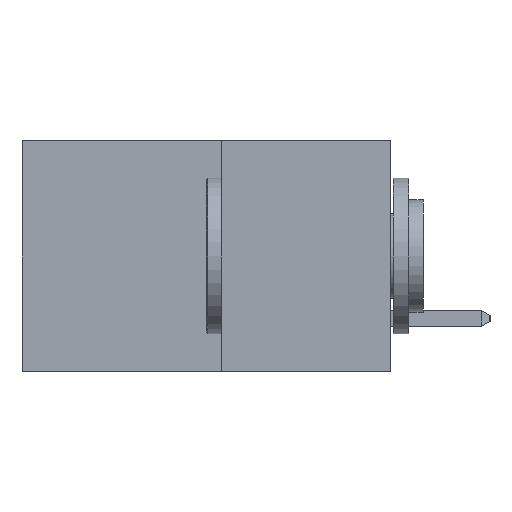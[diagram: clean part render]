
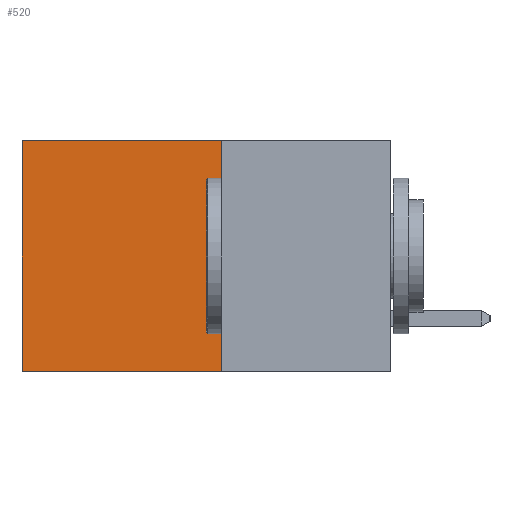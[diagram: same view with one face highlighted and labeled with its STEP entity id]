
A CAD part, left-side view. The second image highlights one B-rep face of the part: STEP entity #520.
In plain terms, the highlighted planar face has unit normal (-1, 0, 0).
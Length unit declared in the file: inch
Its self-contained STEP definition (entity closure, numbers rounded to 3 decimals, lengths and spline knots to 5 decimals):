
#131 = VERTEX_POINT ( 'NONE', #5667 ) ;
#368 = DIRECTION ( 'NONE',  ( 0., 1., 0. ) ) ;
#520 = ADVANCED_FACE ( 'NONE', ( #6625 ), #3044, .F. ) ;
#796 = ORIENTED_EDGE ( 'NONE', *, *, #4600, .F. ) ;
#2286 = DIRECTION ( 'NONE',  ( 0., 0., -1. ) ) ;
#2461 = LINE ( 'NONE', #7073, #4232 ) ;
#2730 = ORIENTED_EDGE ( 'NONE', *, *, #5847, .T. ) ;
#2867 = EDGE_LOOP ( 'NONE', ( #3276, #7098, #796, #2730 ) ) ;
#2904 = VECTOR ( 'NONE', #368, 39.37008 ) ;
#2988 = DIRECTION ( 'NONE',  ( 0., 0., -1. ) ) ;
#3044 = PLANE ( 'NONE',  #6554 ) ;
#3106 = CARTESIAN_POINT ( 'NONE',  ( 0.277, 0.59, 0. ) ) ;
#3276 = ORIENTED_EDGE ( 'NONE', *, *, #8350, .T. ) ;
#3487 = VECTOR ( 'NONE', #8264, 39.37008 ) ;
#4004 = DIRECTION ( 'NONE',  ( 1., 0., 0. ) ) ;
#4232 = VECTOR ( 'NONE', #7167, 39.37008 ) ;
#4600 = EDGE_CURVE ( 'NONE', #131, #5885, #2461, .T. ) ;
#5447 = CARTESIAN_POINT ( 'NONE',  ( 0.277, 0.27, -0.37 ) ) ;
#5470 = CARTESIAN_POINT ( 'NONE',  ( 0.277, 0.59, -0.37 ) ) ;
#5515 = CARTESIAN_POINT ( 'NONE',  ( 0.277, 0.27, -0.37 ) ) ;
#5616 = CARTESIAN_POINT ( 'NONE',  ( 0.277, 0.27, -0.37 ) ) ;
#5667 = CARTESIAN_POINT ( 'NONE',  ( 0.277, 0.27, 0. ) ) ;
#5847 = EDGE_CURVE ( 'NONE', #131, #7130, #6761, .T. ) ;
#5885 = VERTEX_POINT ( 'NONE', #5616 ) ;
#6259 = CARTESIAN_POINT ( 'NONE',  ( 0.277, 0.27, 0. ) ) ;
#6393 = EDGE_CURVE ( 'NONE', #5885, #7320, #9112, .T. ) ;
#6554 = AXIS2_PLACEMENT_3D ( 'NONE', #5515, #4004, #2988 ) ;
#6625 = FACE_OUTER_BOUND ( 'NONE', #2867, .T. ) ;
#6761 = LINE ( 'NONE', #6259, #2904 ) ;
#7012 = LINE ( 'NONE', #7353, #8410 ) ;
#7073 = CARTESIAN_POINT ( 'NONE',  ( 0.277, 0.27, -0.37 ) ) ;
#7098 = ORIENTED_EDGE ( 'NONE', *, *, #6393, .F. ) ;
#7130 = VERTEX_POINT ( 'NONE', #3106 ) ;
#7167 = DIRECTION ( 'NONE',  ( 0., 0., -1. ) ) ;
#7320 = VERTEX_POINT ( 'NONE', #5470 ) ;
#7353 = CARTESIAN_POINT ( 'NONE',  ( 0.277, 0.59, -0.37 ) ) ;
#8264 = DIRECTION ( 'NONE',  ( 0., 1., 0. ) ) ;
#8350 = EDGE_CURVE ( 'NONE', #7130, #7320, #7012, .T. ) ;
#8410 = VECTOR ( 'NONE', #2286, 39.37008 ) ;
#9112 = LINE ( 'NONE', #5447, #3487 ) ;
